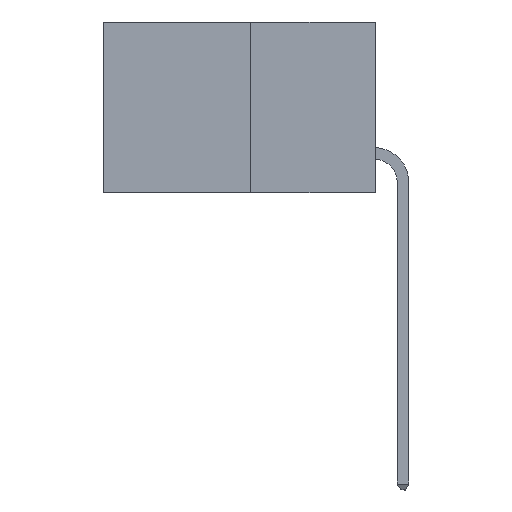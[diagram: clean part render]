
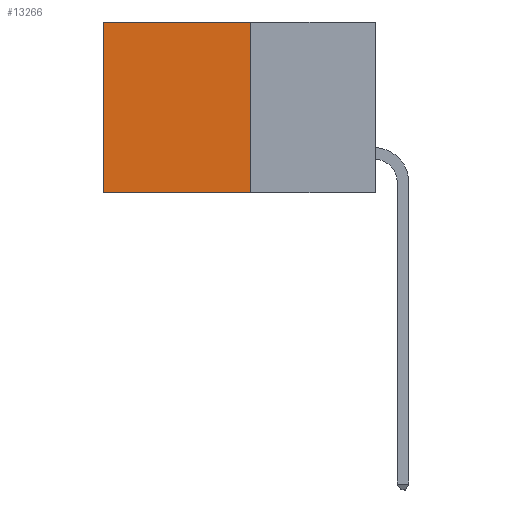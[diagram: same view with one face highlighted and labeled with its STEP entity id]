
A CAD part, left-side view. The second image highlights one B-rep face of the part: STEP entity #13266.
In plain terms, the highlighted planar face has unit normal (-1, 0, 0).
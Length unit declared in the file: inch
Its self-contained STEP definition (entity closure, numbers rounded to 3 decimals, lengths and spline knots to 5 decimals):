
#544 = LINE ( 'NONE', #4366, #4152 ) ;
#1194 = VERTEX_POINT ( 'NONE', #13276 ) ;
#2450 = LINE ( 'NONE', #12531, #5604 ) ;
#3098 = VECTOR ( 'NONE', #5189, 39.37008 ) ;
#3336 = ORIENTED_EDGE ( 'NONE', *, *, #4468, .F. ) ;
#4152 = VECTOR ( 'NONE', #11128, 39.37008 ) ;
#4366 = CARTESIAN_POINT ( 'NONE',  ( 0.277, 0.59, -0.37 ) ) ;
#4468 = EDGE_CURVE ( 'NONE', #16744, #13750, #2450, .T. ) ;
#4622 = EDGE_CURVE ( 'NONE', #5530, #16744, #10305, .T. ) ;
#4650 = EDGE_LOOP ( 'NONE', ( #8892, #3336, #12131, #11524 ) ) ;
#5060 = CARTESIAN_POINT ( 'NONE',  ( 0.277, 0.27, 0. ) ) ;
#5189 = DIRECTION ( 'NONE',  ( 0., 0., -1. ) ) ;
#5530 = VERTEX_POINT ( 'NONE', #12868 ) ;
#5604 = VECTOR ( 'NONE', #9132, 39.37008 ) ;
#6139 = CARTESIAN_POINT ( 'NONE',  ( 0.277, 0.27, -0.37 ) ) ;
#7529 = DIRECTION ( 'NONE',  ( 1., 0., 0. ) ) ;
#7890 = CARTESIAN_POINT ( 'NONE',  ( 0.277, 0.27, -0.37 ) ) ;
#8015 = CARTESIAN_POINT ( 'NONE',  ( 0.277, 0.27, -0.37 ) ) ;
#8487 = EDGE_CURVE ( 'NONE', #1194, #13750, #544, .T. ) ;
#8892 = ORIENTED_EDGE ( 'NONE', *, *, #8487, .T. ) ;
#9132 = DIRECTION ( 'NONE',  ( 0., 1., 0. ) ) ;
#10305 = LINE ( 'NONE', #7890, #3098 ) ;
#11128 = DIRECTION ( 'NONE',  ( 0., 0., -1. ) ) ;
#11524 = ORIENTED_EDGE ( 'NONE', *, *, #16640, .T. ) ;
#12131 = ORIENTED_EDGE ( 'NONE', *, *, #4622, .F. ) ;
#12531 = CARTESIAN_POINT ( 'NONE',  ( 0.277, 0.27, -0.37 ) ) ;
#12868 = CARTESIAN_POINT ( 'NONE',  ( 0.277, 0.27, 0. ) ) ;
#13266 = ADVANCED_FACE ( 'NONE', ( #14802 ), #15645, .F. ) ;
#13276 = CARTESIAN_POINT ( 'NONE',  ( 0.277, 0.59, 0. ) ) ;
#13392 = VECTOR ( 'NONE', #15879, 39.37008 ) ;
#13750 = VERTEX_POINT ( 'NONE', #15328 ) ;
#14802 = FACE_OUTER_BOUND ( 'NONE', #4650, .T. ) ;
#15328 = CARTESIAN_POINT ( 'NONE',  ( 0.277, 0.59, -0.37 ) ) ;
#15645 = PLANE ( 'NONE',  #17353 ) ;
#15879 = DIRECTION ( 'NONE',  ( 0., 1., 0. ) ) ;
#16640 = EDGE_CURVE ( 'NONE', #5530, #1194, #17338, .T. ) ;
#16744 = VERTEX_POINT ( 'NONE', #8015 ) ;
#16919 = DIRECTION ( 'NONE',  ( 0., 0., -1. ) ) ;
#17338 = LINE ( 'NONE', #5060, #13392 ) ;
#17353 = AXIS2_PLACEMENT_3D ( 'NONE', #6139, #7529, #16919 ) ;
